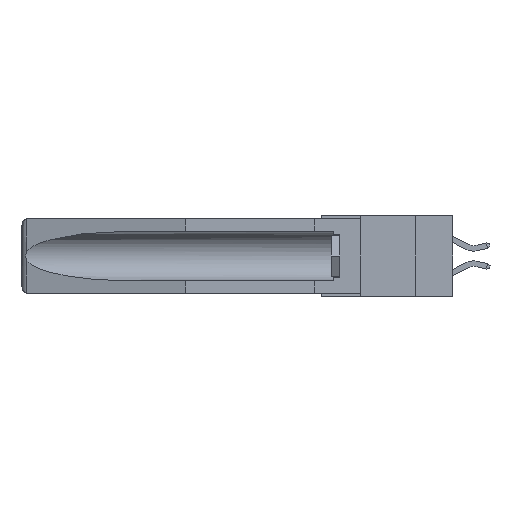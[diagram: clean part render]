
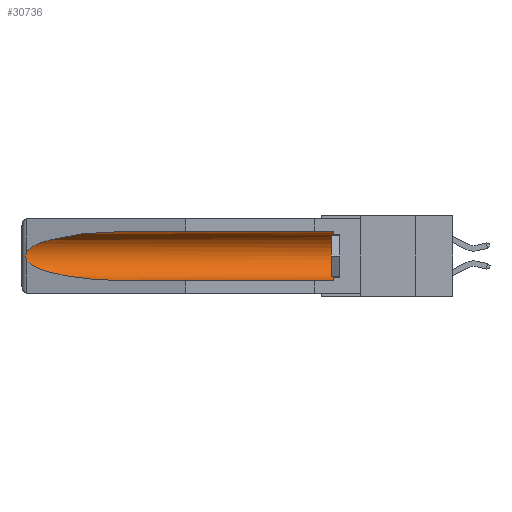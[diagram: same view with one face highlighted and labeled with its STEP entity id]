
A CAD part, left-side view. The second image highlights one B-rep face of the part: STEP entity #30736.
In plain terms, the highlighted cylindrical face has radius 2.857 mm (diameter 5.715 mm), a partial arc.
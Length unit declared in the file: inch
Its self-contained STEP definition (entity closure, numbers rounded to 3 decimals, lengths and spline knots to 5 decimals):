
#258 = EDGE_CURVE ( 'NONE', #27221, #14251, #3337, .T. ) ;
#423 = CARTESIAN_POINT ( 'NONE',  ( 0.26654, 1.53092, -0.15636 ) ) ;
#478 = ORIENTED_EDGE ( 'NONE', *, *, #12903, .T. ) ;
#1539 = CYLINDRICAL_SURFACE ( 'NONE', #7750, 0.1125 ) ;
#1780 = ORIENTED_EDGE ( 'NONE', *, *, #28079, .T. ) ;
#1931 = CARTESIAN_POINT ( 'NONE',  ( 0.155, -0.30754, -0.059 ) ) ;
#1956 = EDGE_CURVE ( 'NONE', #27283, #28867, #28045, .T. ) ;
#2143 = VECTOR ( 'NONE', #10406, 39.37008 ) ;
#2433 = DIRECTION ( 'NONE',  ( 0., 1., 0. ) ) ;
#2618 = VERTEX_POINT ( 'NONE', #14211 ) ;
#2635 = CARTESIAN_POINT ( 'NONE',  ( 0.2673, 1.53269, -0.17917 ) ) ;
#3337 =( BOUNDED_CURVE ( )  B_SPLINE_CURVE ( 3, ( #20238, #25296, #10419, #12920 ),
 .UNSPECIFIED., .F., .F. ) 
 B_SPLINE_CURVE_WITH_KNOTS ( ( 4, 4 ),
 ( 0.1948, 1.5708 ),
 .UNSPECIFIED. ) 
 CURVE ( )  GEOMETRIC_REPRESENTATION_ITEM ( )  RATIONAL_B_SPLINE_CURVE ( ( 1., 0.848, 0.848, 1. ) ) 
 REPRESENTATION_ITEM ( '' )  );
#4924 = DIRECTION ( 'NONE',  ( 0., 0., 1. ) ) ;
#5120 = CARTESIAN_POINT ( 'NONE',  ( 0.26597, 1.5296, -0.19026 ) ) ;
#5328 = CARTESIAN_POINT ( 'NONE',  ( 0.155, 1.07973, -0.059 ) ) ;
#7095 = ORIENTED_EDGE ( 'NONE', *, *, #1956, .T. ) ;
#7750 = AXIS2_PLACEMENT_3D ( 'NONE', #24427, #2433, #4924 ) ;
#9032 = AXIS2_PLACEMENT_3D ( 'NONE', #17504, #15241, #12668 ) ;
#9915 = ORIENTED_EDGE ( 'NONE', *, *, #22902, .F. ) ;
#10406 = DIRECTION ( 'NONE',  ( 0., 1., 0. ) ) ;
#10419 = CARTESIAN_POINT ( 'NONE',  ( 0.21114, 1.30732, -0.284 ) ) ;
#10467 =( BOUNDED_CURVE ( )  B_SPLINE_CURVE ( 3, ( #5328, #27446, #12686, #32136 ),
 .UNSPECIFIED., .F., .F. ) 
 B_SPLINE_CURVE_WITH_KNOTS ( ( 4, 4 ),
 ( 4.71239, 6.08839 ),
 .UNSPECIFIED. ) 
 CURVE ( )  GEOMETRIC_REPRESENTATION_ITEM ( )  RATIONAL_B_SPLINE_CURVE ( ( 1., 0.848, 0.848, 1. ) ) 
 REPRESENTATION_ITEM ( '' )  );
#11062 = CARTESIAN_POINT ( 'NONE',  ( 0.155, 1.07973, -0.284 ) ) ;
#11235 = FACE_OUTER_BOUND ( 'NONE', #20687, .T. ) ;
#11953 = CIRCLE ( 'NONE', #9032, 0.1125 ) ;
#12668 = DIRECTION ( 'NONE',  ( 0., 0., 1. ) ) ;
#12686 = CARTESIAN_POINT ( 'NONE',  ( 0.25451, 1.48313, -0.09465 ) ) ;
#12806 = CARTESIAN_POINT ( 'NONE',  ( 0.2675, 1.53308, -0.17534 ) ) ;
#12903 = EDGE_CURVE ( 'NONE', #28867, #17592, #10467, .T. ) ;
#12920 = CARTESIAN_POINT ( 'NONE',  ( 0.155, 1.07973, -0.284 ) ) ;
#13137 = CARTESIAN_POINT ( 'NONE',  ( 0.26537, 1.52718, -0.19328 ) ) ;
#14211 = CARTESIAN_POINT ( 'NONE',  ( 0.155, 0.126, -0.284 ) ) ;
#14251 = VERTEX_POINT ( 'NONE', #11062 ) ;
#14865 = CARTESIAN_POINT ( 'NONE',  ( 0.26655, 1.53094, -0.18657 ) ) ;
#15067 = CARTESIAN_POINT ( 'NONE',  ( 0.155, -0.30754, -0.284 ) ) ;
#15166 = CARTESIAN_POINT ( 'NONE',  ( 0.26537, 1.52718, -0.19328 ) ) ;
#15241 = DIRECTION ( 'NONE',  ( 0., -1., 0. ) ) ;
#17504 = CARTESIAN_POINT ( 'NONE',  ( 0.155, 0.126, -0.1715 ) ) ;
#17592 = VERTEX_POINT ( 'NONE', #23544 ) ;
#19814 = CARTESIAN_POINT ( 'NONE',  ( 0.2673, 1.5327, -0.16383 ) ) ;
#20238 = CARTESIAN_POINT ( 'NONE',  ( 0.26537, 1.52718, -0.19328 ) ) ;
#20687 = EDGE_LOOP ( 'NONE', ( #478, #1780, #28583, #9915, #22232, #7095 ) ) ;
#21459 = EDGE_CURVE ( 'NONE', #2618, #27283, #11953, .T. ) ;
#22232 = ORIENTED_EDGE ( 'NONE', *, *, #21459, .T. ) ;
#22902 = EDGE_CURVE ( 'NONE', #2618, #14251, #23454, .T. ) ;
#23454 = LINE ( 'NONE', #15067, #2143 ) ;
#23544 = CARTESIAN_POINT ( 'NONE',  ( 0.26537, 1.52718, -0.14972 ) ) ;
#24427 = CARTESIAN_POINT ( 'NONE',  ( 0.155, -0.30754, -0.1715 ) ) ;
#24951 = CARTESIAN_POINT ( 'NONE',  ( 0.26537, 1.52718, -0.14972 ) ) ;
#25296 = CARTESIAN_POINT ( 'NONE',  ( 0.25451, 1.48313, -0.24835 ) ) ;
#27221 = VERTEX_POINT ( 'NONE', #13137 ) ;
#27283 = VERTEX_POINT ( 'NONE', #31371 ) ;
#27446 = CARTESIAN_POINT ( 'NONE',  ( 0.21114, 1.30732, -0.059 ) ) ;
#27459 = CARTESIAN_POINT ( 'NONE',  ( 0.2675, 1.53308, -0.16763 ) ) ;
#28045 = LINE ( 'NONE', #1931, #31538 ) ;
#28079 = EDGE_CURVE ( 'NONE', #17592, #27221, #29816, .T. ) ;
#28583 = ORIENTED_EDGE ( 'NONE', *, *, #258, .T. ) ;
#28867 = VERTEX_POINT ( 'NONE', #30433 ) ;
#29188 = DIRECTION ( 'NONE',  ( 0., 1., 0. ) ) ;
#29816 = B_SPLINE_CURVE_WITH_KNOTS ( 'NONE', 3,
 ( #24951, #30185, #423, #19814, #27459, #12806, #2635, #14865, #5120, #15166 ),
 .UNSPECIFIED., .F., .F.,
 ( 4, 2, 2, 2, 4 ),
 ( 0., 0.00029, 0.00058, 0.00087, 0.00117 ),
 .UNSPECIFIED. ) ;
#30185 = CARTESIAN_POINT ( 'NONE',  ( 0.26597, 1.52961, -0.15275 ) ) ;
#30433 = CARTESIAN_POINT ( 'NONE',  ( 0.155, 1.07973, -0.059 ) ) ;
#30736 = ADVANCED_FACE ( 'NONE', ( #11235 ), #1539, .F. ) ;
#31371 = CARTESIAN_POINT ( 'NONE',  ( 0.155, 0.126, -0.059 ) ) ;
#31538 = VECTOR ( 'NONE', #29188, 39.37008 ) ;
#32136 = CARTESIAN_POINT ( 'NONE',  ( 0.26537, 1.52718, -0.14972 ) ) ;
